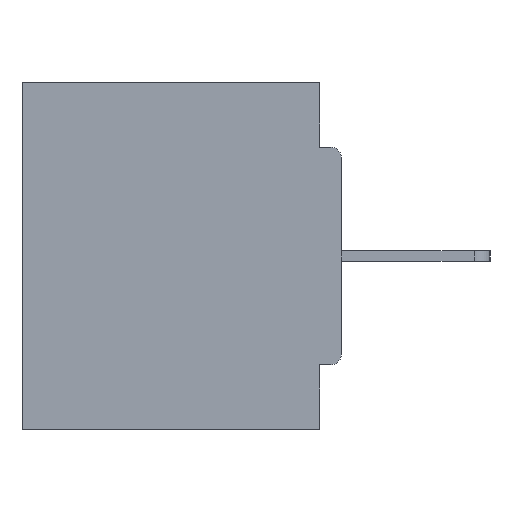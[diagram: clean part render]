
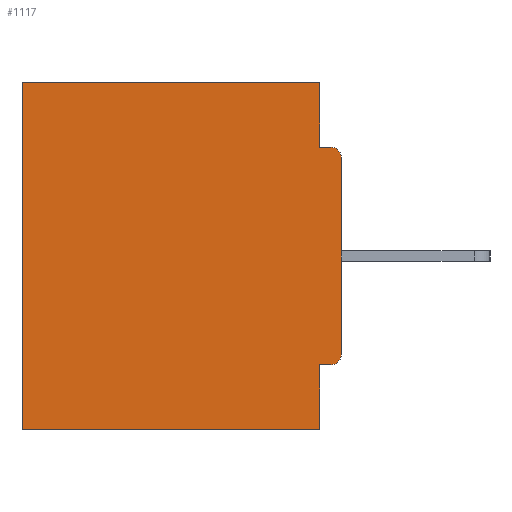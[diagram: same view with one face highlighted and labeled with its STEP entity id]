
A CAD part, left-side view. The second image highlights one B-rep face of the part: STEP entity #1117.
In plain terms, the highlighted planar face has unit normal (-1, 0, 0).
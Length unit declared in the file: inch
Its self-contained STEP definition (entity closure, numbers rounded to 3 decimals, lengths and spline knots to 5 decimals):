
#527 = DIRECTION ( 'NONE',  ( 1., 0., 0. ) ) ;
#793 = DIRECTION ( 'NONE',  ( 0., 0., -1. ) ) ;
#1107 = CARTESIAN_POINT ( 'NONE',  ( 0.298, 0.031, -0.4065 ) ) ;
#1117 = ADVANCED_FACE ( 'NONE', ( #11240 ), #2227, .F. ) ;
#1598 = VECTOR ( 'NONE', #12164, 39.37008 ) ;
#1858 = LINE ( 'NONE', #12882, #21706 ) ;
#2227 = PLANE ( 'NONE',  #26123 ) ;
#2619 = CARTESIAN_POINT ( 'NONE',  ( 0.298, 0.46, -0.5 ) ) ;
#2991 = VERTEX_POINT ( 'NONE', #16048 ) ;
#4150 = EDGE_CURVE ( 'NONE', #22288, #24639, #15962, .T. ) ;
#4381 = CIRCLE ( 'NONE', #16376, 0.015 ) ;
#6052 = ORIENTED_EDGE ( 'NONE', *, *, #22034, .F. ) ;
#6094 = EDGE_CURVE ( 'NONE', #2991, #22288, #15860, .T. ) ;
#6315 = VECTOR ( 'NONE', #26865, 39.37008 ) ;
#6645 = LINE ( 'NONE', #14085, #20195 ) ;
#6828 = ORIENTED_EDGE ( 'NONE', *, *, #34318, .T. ) ;
#7346 = CARTESIAN_POINT ( 'NONE',  ( 0.298, 0.031, -0.5 ) ) ;
#7347 = VERTEX_POINT ( 'NONE', #30317 ) ;
#8117 = ORIENTED_EDGE ( 'NONE', *, *, #11964, .F. ) ;
#9070 = VERTEX_POINT ( 'NONE', #13113 ) ;
#9496 = VECTOR ( 'NONE', #11510, 39.37008 ) ;
#10538 = ORIENTED_EDGE ( 'NONE', *, *, #6094, .F. ) ;
#10634 = CARTESIAN_POINT ( 'NONE',  ( 0.298, 0.031, -0.5 ) ) ;
#10762 = ORIENTED_EDGE ( 'NONE', *, *, #14175, .T. ) ;
#11080 = CARTESIAN_POINT ( 'NONE',  ( 0.298, 0.015, -0.3915 ) ) ;
#11240 = FACE_OUTER_BOUND ( 'NONE', #13419, .T. ) ;
#11510 = DIRECTION ( 'NONE',  ( 0., 1., 0. ) ) ;
#11964 = EDGE_CURVE ( 'NONE', #23272, #30227, #1858, .T. ) ;
#12164 = DIRECTION ( 'NONE',  ( 0., 0., -1. ) ) ;
#12196 = DIRECTION ( 'NONE',  ( -1., 0., 0. ) ) ;
#12591 = ORIENTED_EDGE ( 'NONE', *, *, #4150, .F. ) ;
#12882 = CARTESIAN_POINT ( 'NONE',  ( 0.298, 0., -0.0935 ) ) ;
#12889 = EDGE_CURVE ( 'NONE', #17337, #17525, #28439, .T. ) ;
#13113 = CARTESIAN_POINT ( 'NONE',  ( 0.298, 0.46, 0. ) ) ;
#13419 = EDGE_LOOP ( 'NONE', ( #14393, #8117, #6052, #10762, #6828, #29911, #12591, #10538, #29668, #15819 ) ) ;
#13499 = LINE ( 'NONE', #10634, #6315 ) ;
#13831 = DIRECTION ( 'NONE',  ( 0., 0., -1. ) ) ;
#14085 = CARTESIAN_POINT ( 'NONE',  ( 0.298, 0., -0.5 ) ) ;
#14175 = EDGE_CURVE ( 'NONE', #7347, #9070, #28342, .T. ) ;
#14393 = ORIENTED_EDGE ( 'NONE', *, *, #25645, .T. ) ;
#14704 = VECTOR ( 'NONE', #19405, 39.37008 ) ;
#15538 = LINE ( 'NONE', #24719, #14704 ) ;
#15819 = ORIENTED_EDGE ( 'NONE', *, *, #12889, .F. ) ;
#15860 = LINE ( 'NONE', #20688, #9496 ) ;
#15962 = LINE ( 'NONE', #24590, #1598 ) ;
#16048 = CARTESIAN_POINT ( 'NONE',  ( 0.298, 0.015, -0.4065 ) ) ;
#16373 = VERTEX_POINT ( 'NONE', #2619 ) ;
#16376 = AXIS2_PLACEMENT_3D ( 'NONE', #28408, #12196, #31071 ) ;
#16813 = DIRECTION ( 'NONE',  ( 0., 1., 0. ) ) ;
#17337 = VERTEX_POINT ( 'NONE', #31603 ) ;
#17525 = VERTEX_POINT ( 'NONE', #21765 ) ;
#19405 = DIRECTION ( 'NONE',  ( 0., 0., -1. ) ) ;
#19577 = VECTOR ( 'NONE', #24910, 39.37008 ) ;
#20195 = VECTOR ( 'NONE', #16813, 39.37008 ) ;
#20688 = CARTESIAN_POINT ( 'NONE',  ( 0.298, 0., -0.4065 ) ) ;
#21154 = VECTOR ( 'NONE', #31957, 39.37008 ) ;
#21706 = VECTOR ( 'NONE', #23799, 39.37008 ) ;
#21765 = CARTESIAN_POINT ( 'NONE',  ( 0.298, 0., -0.3915 ) ) ;
#22016 = CARTESIAN_POINT ( 'NONE',  ( 0.298, 0.015, -0.0935 ) ) ;
#22034 = EDGE_CURVE ( 'NONE', #7347, #23272, #13499, .T. ) ;
#22288 = VERTEX_POINT ( 'NONE', #1107 ) ;
#23272 = VERTEX_POINT ( 'NONE', #32006 ) ;
#23786 = CARTESIAN_POINT ( 'NONE',  ( 0.298, 0., 0. ) ) ;
#23799 = DIRECTION ( 'NONE',  ( 0., -1., 0. ) ) ;
#24590 = CARTESIAN_POINT ( 'NONE',  ( 0.298, 0.031, -0.5 ) ) ;
#24639 = VERTEX_POINT ( 'NONE', #7346 ) ;
#24719 = CARTESIAN_POINT ( 'NONE',  ( 0.298, 0.46, 0. ) ) ;
#24910 = DIRECTION ( 'NONE',  ( 0., 0., -1. ) ) ;
#25152 = CARTESIAN_POINT ( 'NONE',  ( 0.298, 0., 0. ) ) ;
#25190 = AXIS2_PLACEMENT_3D ( 'NONE', #11080, #29985, #13831 ) ;
#25645 = EDGE_CURVE ( 'NONE', #17337, #30227, #4381, .T. ) ;
#26123 = AXIS2_PLACEMENT_3D ( 'NONE', #25152, #527, #793 ) ;
#26639 = EDGE_CURVE ( 'NONE', #2991, #17525, #28771, .T. ) ;
#26865 = DIRECTION ( 'NONE',  ( 0., 0., -1. ) ) ;
#27650 = CARTESIAN_POINT ( 'NONE',  ( 0.298, 0., 0. ) ) ;
#28342 = LINE ( 'NONE', #23786, #21154 ) ;
#28408 = CARTESIAN_POINT ( 'NONE',  ( 0.298, 0.015, -0.1085 ) ) ;
#28439 = LINE ( 'NONE', #27650, #19577 ) ;
#28771 = CIRCLE ( 'NONE', #25190, 0.015 ) ;
#29668 = ORIENTED_EDGE ( 'NONE', *, *, #26639, .T. ) ;
#29911 = ORIENTED_EDGE ( 'NONE', *, *, #34354, .F. ) ;
#29985 = DIRECTION ( 'NONE',  ( -1., 0., 0. ) ) ;
#30227 = VERTEX_POINT ( 'NONE', #22016 ) ;
#30317 = CARTESIAN_POINT ( 'NONE',  ( 0.298, 0.031, 0. ) ) ;
#31071 = DIRECTION ( 'NONE',  ( 0., 0., -1. ) ) ;
#31603 = CARTESIAN_POINT ( 'NONE',  ( 0.298, 0., -0.1085 ) ) ;
#31957 = DIRECTION ( 'NONE',  ( 0., 1., 0. ) ) ;
#32006 = CARTESIAN_POINT ( 'NONE',  ( 0.298, 0.031, -0.0935 ) ) ;
#34318 = EDGE_CURVE ( 'NONE', #9070, #16373, #15538, .T. ) ;
#34354 = EDGE_CURVE ( 'NONE', #24639, #16373, #6645, .T. ) ;
